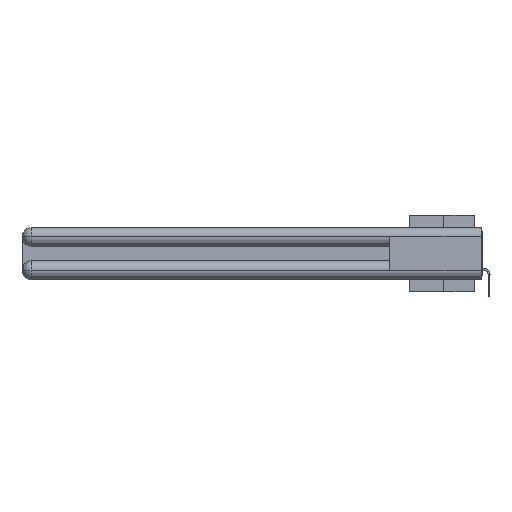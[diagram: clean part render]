
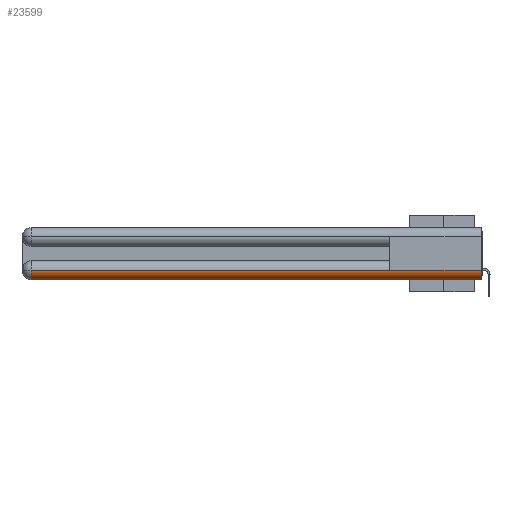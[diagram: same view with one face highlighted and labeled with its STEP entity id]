
A CAD part, left-side view. The second image highlights one B-rep face of the part: STEP entity #23599.
In plain terms, the highlighted cylindrical face has radius 1.562 mm (diameter 3.124 mm), a partial arc.
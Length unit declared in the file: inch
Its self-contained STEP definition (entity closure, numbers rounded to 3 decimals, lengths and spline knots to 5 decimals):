
#291 = EDGE_CURVE ( 'NONE', #5633, #21817, #4163, .T. ) ;
#1234 = EDGE_CURVE ( 'NONE', #21817, #7734, #29067, .T. ) ;
#1275 = DIRECTION ( 'NONE',  ( 0., 0., -1. ) ) ;
#2017 = VECTOR ( 'NONE', #23232, 39.37008 ) ;
#3447 = AXIS2_PLACEMENT_3D ( 'NONE', #26125, #23553, #1275 ) ;
#3575 = AXIS2_PLACEMENT_3D ( 'NONE', #22168, #17268, #33586 ) ;
#3997 = FACE_OUTER_BOUND ( 'NONE', #32871, .T. ) ;
#4163 = LINE ( 'NONE', #17423, #15004 ) ;
#5633 = VERTEX_POINT ( 'NONE', #13082 ) ;
#6245 = ORIENTED_EDGE ( 'NONE', *, *, #16461, .F. ) ;
#6717 = DIRECTION ( 'NONE',  ( 0., 1., 0. ) ) ;
#7114 = CARTESIAN_POINT ( 'NONE',  ( 0., 2.94, -0.2785 ) ) ;
#7452 = LINE ( 'NONE', #12185, #2017 ) ;
#7734 = VERTEX_POINT ( 'NONE', #22621 ) ;
#8302 = AXIS2_PLACEMENT_3D ( 'NONE', #29669, #35106, #10455 ) ;
#10455 = DIRECTION ( 'NONE',  ( 1., 0., 0. ) ) ;
#12135 = CARTESIAN_POINT ( 'NONE',  ( 0.0615, 0., -0.34 ) ) ;
#12185 = CARTESIAN_POINT ( 'NONE',  ( 0., 0., -0.2785 ) ) ;
#12937 = ORIENTED_EDGE ( 'NONE', *, *, #291, .T. ) ;
#13082 = CARTESIAN_POINT ( 'NONE',  ( 0., 0.6, -0.2785 ) ) ;
#14096 = CIRCLE ( 'NONE', #8302, 0.0615 ) ;
#15004 = VECTOR ( 'NONE', #6717, 39.37008 ) ;
#15068 = CYLINDRICAL_SURFACE ( 'NONE', #3447, 0.0615 ) ;
#16461 = EDGE_CURVE ( 'NONE', #5633, #18352, #7452, .T. ) ;
#17268 = DIRECTION ( 'NONE',  ( 0., -1., 0. ) ) ;
#17423 = CARTESIAN_POINT ( 'NONE',  ( 0., 0., -0.2785 ) ) ;
#17435 = ORIENTED_EDGE ( 'NONE', *, *, #30298, .F. ) ;
#17505 = DIRECTION ( 'NONE',  ( 0., 1., 0. ) ) ;
#18352 = VERTEX_POINT ( 'NONE', #33525 ) ;
#18451 = VERTEX_POINT ( 'NONE', #12135 ) ;
#18908 = ORIENTED_EDGE ( 'NONE', *, *, #23160, .F. ) ;
#19710 = VECTOR ( 'NONE', #17505, 39.37008 ) ;
#21817 = VERTEX_POINT ( 'NONE', #7114 ) ;
#22168 = CARTESIAN_POINT ( 'NONE',  ( 0.0615, 2.94, -0.2785 ) ) ;
#22621 = CARTESIAN_POINT ( 'NONE',  ( 0.0615, 2.94, -0.34 ) ) ;
#23160 = EDGE_CURVE ( 'NONE', #18451, #7734, #35018, .T. ) ;
#23232 = DIRECTION ( 'NONE',  ( 0., -1., 0. ) ) ;
#23553 = DIRECTION ( 'NONE',  ( 0., -1., 0. ) ) ;
#23599 = ADVANCED_FACE ( 'NONE', ( #3997 ), #15068, .T. ) ;
#23774 = CARTESIAN_POINT ( 'NONE',  ( 0.0615, 0., -0.34 ) ) ;
#26125 = CARTESIAN_POINT ( 'NONE',  ( 0.0615, 0., -0.2785 ) ) ;
#29067 = CIRCLE ( 'NONE', #3575, 0.0615 ) ;
#29669 = CARTESIAN_POINT ( 'NONE',  ( 0.0615, 0., -0.2785 ) ) ;
#29979 = ORIENTED_EDGE ( 'NONE', *, *, #1234, .T. ) ;
#30298 = EDGE_CURVE ( 'NONE', #18352, #18451, #14096, .T. ) ;
#32871 = EDGE_LOOP ( 'NONE', ( #12937, #29979, #18908, #17435, #6245 ) ) ;
#33525 = CARTESIAN_POINT ( 'NONE',  ( 0., 0., -0.2785 ) ) ;
#33586 = DIRECTION ( 'NONE',  ( 0., 0., 1. ) ) ;
#35018 = LINE ( 'NONE', #23774, #19710 ) ;
#35106 = DIRECTION ( 'NONE',  ( 0., -1., 0. ) ) ;
